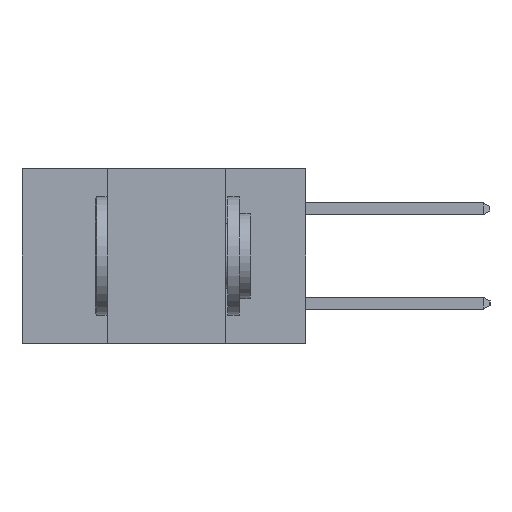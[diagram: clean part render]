
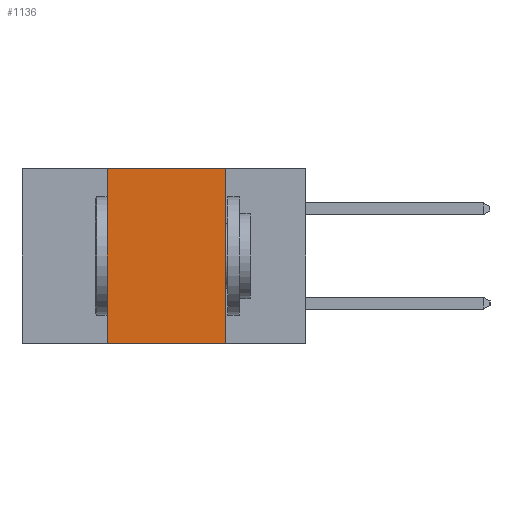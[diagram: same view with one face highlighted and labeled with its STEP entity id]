
A CAD part, left-side view. The second image highlights one B-rep face of the part: STEP entity #1136.
In plain terms, the highlighted planar face has unit normal (-1, 0, 0).
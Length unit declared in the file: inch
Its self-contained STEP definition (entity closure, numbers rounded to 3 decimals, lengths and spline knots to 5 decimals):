
#1136 = ADVANCED_FACE ( 'NONE', ( #9531 ), #10678, .F. ) ;
#2620 = ORIENTED_EDGE ( 'NONE', *, *, #12121, .F. ) ;
#2852 = CARTESIAN_POINT ( 'NONE',  ( 0., 0.17, 0. ) ) ;
#2987 = VERTEX_POINT ( 'NONE', #3450 ) ;
#3363 = LINE ( 'NONE', #6764, #5133 ) ;
#3450 = CARTESIAN_POINT ( 'NONE',  ( 0., 0.42, -0.37 ) ) ;
#3601 = CARTESIAN_POINT ( 'NONE',  ( 0., 0.6, -0.37 ) ) ;
#3860 = VECTOR ( 'NONE', #8332, 39.37008 ) ;
#4112 = VECTOR ( 'NONE', #11445, 39.37008 ) ;
#4157 = CARTESIAN_POINT ( 'NONE',  ( 0., 0.42, 0. ) ) ;
#4490 = EDGE_CURVE ( 'NONE', #2987, #13402, #6678, .T. ) ;
#4967 = ORIENTED_EDGE ( 'NONE', *, *, #6274, .F. ) ;
#5098 = CARTESIAN_POINT ( 'NONE',  ( 0., 0.42, -0.37 ) ) ;
#5133 = VECTOR ( 'NONE', #6725, 39.37008 ) ;
#6274 = EDGE_CURVE ( 'NONE', #6557, #13402, #3363, .T. ) ;
#6557 = VERTEX_POINT ( 'NONE', #2852 ) ;
#6678 = LINE ( 'NONE', #3601, #3860 ) ;
#6725 = DIRECTION ( 'NONE',  ( 0., 0., -1. ) ) ;
#6764 = CARTESIAN_POINT ( 'NONE',  ( 0., 0.17, -0.37 ) ) ;
#6785 = VECTOR ( 'NONE', #9216, 39.37008 ) ;
#6933 = LINE ( 'NONE', #5098, #4112 ) ;
#7167 = ORIENTED_EDGE ( 'NONE', *, *, #12789, .F. ) ;
#7568 = EDGE_LOOP ( 'NONE', ( #4967, #2620, #7167, #7752 ) ) ;
#7660 = VERTEX_POINT ( 'NONE', #4157 ) ;
#7752 = ORIENTED_EDGE ( 'NONE', *, *, #4490, .T. ) ;
#8332 = DIRECTION ( 'NONE',  ( 0., -1., 0. ) ) ;
#9216 = DIRECTION ( 'NONE',  ( 0., -1., 0. ) ) ;
#9405 = CARTESIAN_POINT ( 'NONE',  ( 0., 0.6, 0. ) ) ;
#9531 = FACE_OUTER_BOUND ( 'NONE', #7568, .T. ) ;
#9559 = LINE ( 'NONE', #9405, #6785 ) ;
#9988 = DIRECTION ( 'NONE',  ( 0., 0., -1. ) ) ;
#10184 = DIRECTION ( 'NONE',  ( 1., 0., 0. ) ) ;
#10392 = CARTESIAN_POINT ( 'NONE',  ( 0., 0.17, -0.37 ) ) ;
#10488 = AXIS2_PLACEMENT_3D ( 'NONE', #12587, #10184, #9988 ) ;
#10678 = PLANE ( 'NONE',  #10488 ) ;
#11445 = DIRECTION ( 'NONE',  ( 0., 0., 1. ) ) ;
#12121 = EDGE_CURVE ( 'NONE', #7660, #6557, #9559, .T. ) ;
#12587 = CARTESIAN_POINT ( 'NONE',  ( 0., 0.6, 0. ) ) ;
#12789 = EDGE_CURVE ( 'NONE', #2987, #7660, #6933, .T. ) ;
#13402 = VERTEX_POINT ( 'NONE', #10392 ) ;
